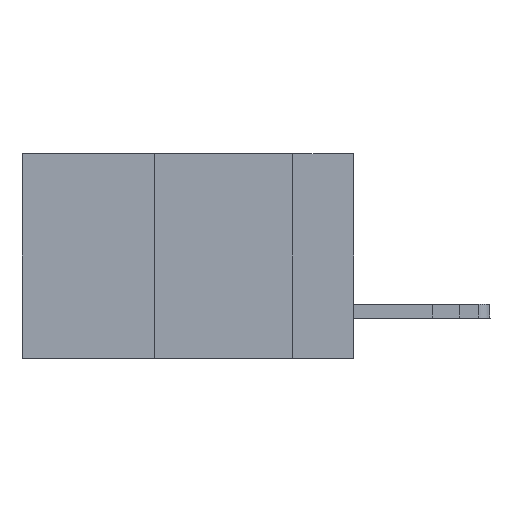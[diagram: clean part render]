
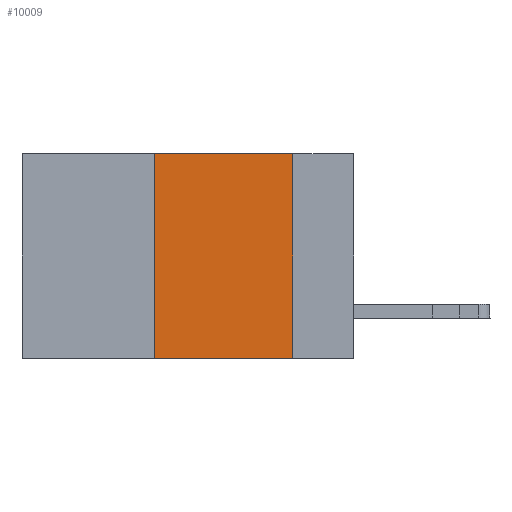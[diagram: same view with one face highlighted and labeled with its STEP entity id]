
A CAD part, left-side view. The second image highlights one B-rep face of the part: STEP entity #10009.
In plain terms, the highlighted planar face has unit normal (-1, 0, 0).
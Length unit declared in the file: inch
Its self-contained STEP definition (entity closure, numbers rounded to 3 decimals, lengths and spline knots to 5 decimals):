
#534 = VERTEX_POINT ( 'NONE', #17952 ) ;
#1535 = VERTEX_POINT ( 'NONE', #15144 ) ;
#3712 = CARTESIAN_POINT ( 'NONE',  ( 0., 0.36, -0.37 ) ) ;
#4314 = FACE_OUTER_BOUND ( 'NONE', #17164, .T. ) ;
#4458 = DIRECTION ( 'NONE',  ( 0., -1., 0. ) ) ;
#5253 = ORIENTED_EDGE ( 'NONE', *, *, #18252, .F. ) ;
#6445 = LINE ( 'NONE', #11578, #19212 ) ;
#6627 = DIRECTION ( 'NONE',  ( 0., 0., -1. ) ) ;
#6771 = DIRECTION ( 'NONE',  ( 0., -1., 0. ) ) ;
#7499 = VECTOR ( 'NONE', #10300, 39.37008 ) ;
#7767 = VERTEX_POINT ( 'NONE', #24077 ) ;
#7768 = ORIENTED_EDGE ( 'NONE', *, *, #24728, .T. ) ;
#9436 = PLANE ( 'NONE',  #17392 ) ;
#10009 = ADVANCED_FACE ( 'NONE', ( #4314 ), #9436, .F. ) ;
#10300 = DIRECTION ( 'NONE',  ( 0., 0., 1. ) ) ;
#11493 = EDGE_CURVE ( 'NONE', #534, #1535, #17839, .T. ) ;
#11578 = CARTESIAN_POINT ( 'NONE',  ( 0., 0.6, -0.37 ) ) ;
#11911 = DIRECTION ( 'NONE',  ( 1., 0., 0. ) ) ;
#12814 = EDGE_CURVE ( 'NONE', #24298, #7767, #15073, .T. ) ;
#15073 = LINE ( 'NONE', #22692, #7499 ) ;
#15144 = CARTESIAN_POINT ( 'NONE',  ( 0., 0.11, -0.37 ) ) ;
#17008 = LINE ( 'NONE', #22463, #29853 ) ;
#17164 = EDGE_LOOP ( 'NONE', ( #22693, #5253, #27362, #7768 ) ) ;
#17392 = AXIS2_PLACEMENT_3D ( 'NONE', #32425, #11911, #6627 ) ;
#17839 = LINE ( 'NONE', #28106, #26477 ) ;
#17952 = CARTESIAN_POINT ( 'NONE',  ( 0., 0.11, 0. ) ) ;
#18252 = EDGE_CURVE ( 'NONE', #7767, #534, #17008, .T. ) ;
#19212 = VECTOR ( 'NONE', #6771, 39.37008 ) ;
#22463 = CARTESIAN_POINT ( 'NONE',  ( 0., 0.6, 0. ) ) ;
#22692 = CARTESIAN_POINT ( 'NONE',  ( 0., 0.36, 0. ) ) ;
#22693 = ORIENTED_EDGE ( 'NONE', *, *, #11493, .F. ) ;
#24077 = CARTESIAN_POINT ( 'NONE',  ( 0., 0.36, 0. ) ) ;
#24298 = VERTEX_POINT ( 'NONE', #3712 ) ;
#24728 = EDGE_CURVE ( 'NONE', #24298, #1535, #6445, .T. ) ;
#26477 = VECTOR ( 'NONE', #27777, 39.37008 ) ;
#27362 = ORIENTED_EDGE ( 'NONE', *, *, #12814, .F. ) ;
#27777 = DIRECTION ( 'NONE',  ( 0., 0., -1. ) ) ;
#28106 = CARTESIAN_POINT ( 'NONE',  ( 0., 0.11, 0. ) ) ;
#29853 = VECTOR ( 'NONE', #4458, 39.37008 ) ;
#32425 = CARTESIAN_POINT ( 'NONE',  ( 0., 0.6, 0. ) ) ;
